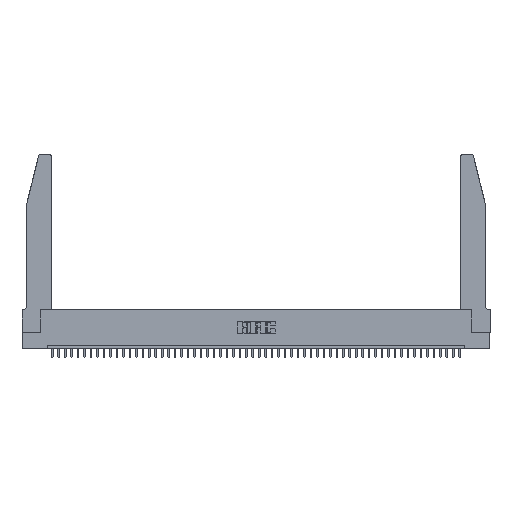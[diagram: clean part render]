
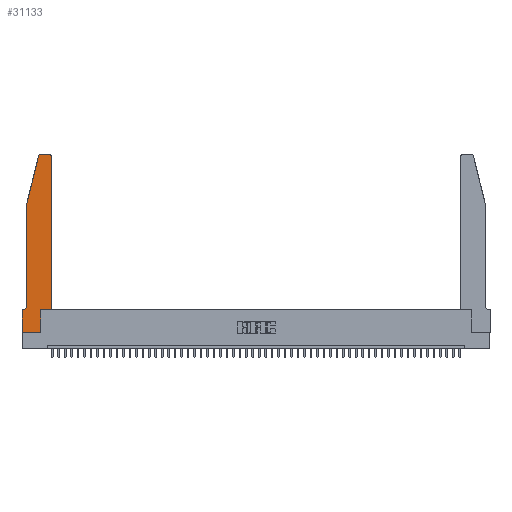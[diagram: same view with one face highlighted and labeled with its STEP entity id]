
A CAD part, top view. The second image highlights one B-rep face of the part: STEP entity #31133.
In plain terms, the highlighted planar face has unit normal (0, 0, 1).
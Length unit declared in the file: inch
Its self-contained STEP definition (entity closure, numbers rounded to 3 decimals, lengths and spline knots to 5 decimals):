
#1717 = ORIENTED_EDGE ( 'NONE', *, *, #28903, .T. ) ;
#1840 = EDGE_CURVE ( 'NONE', #20062, #29995, #32246, .T. ) ;
#2318 = CARTESIAN_POINT ( 'NONE',  ( 0.0055, 0.35, 0.37 ) ) ;
#3267 = CARTESIAN_POINT ( 'NONE',  ( 0.284, 2.75, 0.37 ) ) ;
#3739 = VERTEX_POINT ( 'NONE', #6197 ) ;
#4119 = EDGE_CURVE ( 'NONE', #8806, #45292, #38671, .T. ) ;
#4147 = ORIENTED_EDGE ( 'NONE', *, *, #32344, .T. ) ;
#6197 = CARTESIAN_POINT ( 'NONE',  ( 0., 0.35, 0.37 ) ) ;
#6241 = CARTESIAN_POINT ( 'NONE',  ( 0.25487, 2.72718, 0.37 ) ) ;
#6331 = CARTESIAN_POINT ( 'NONE',  ( 0.4505, 0.35, 0.37 ) ) ;
#6608 = ORIENTED_EDGE ( 'NONE', *, *, #1840, .T. ) ;
#6684 = DIRECTION ( 'NONE',  ( 1., 0., 0. ) ) ;
#6787 = CARTESIAN_POINT ( 'NONE',  ( 0.2605, 2.75, 0.37 ) ) ;
#7058 = CARTESIAN_POINT ( 'NONE',  ( 0.0755, 2., 0.37 ) ) ;
#7132 = AXIS2_PLACEMENT_3D ( 'NONE', #12998, #8782, #47065 ) ;
#7313 = CARTESIAN_POINT ( 'NONE',  ( 0.0755, 2., 0.37 ) ) ;
#7950 = VERTEX_POINT ( 'NONE', #2318 ) ;
#8351 = EDGE_CURVE ( 'NONE', #29320, #8806, #15928, .T. ) ;
#8782 = DIRECTION ( 'NONE',  ( 0., 0., 1. ) ) ;
#8806 = VERTEX_POINT ( 'NONE', #7058 ) ;
#8993 = VERTEX_POINT ( 'NONE', #33100 ) ;
#9275 = CIRCLE ( 'NONE', #34015, 0.07 ) ;
#9447 = CARTESIAN_POINT ( 'NONE',  ( 0.2865, 0., 0.37 ) ) ;
#9483 = VERTEX_POINT ( 'NONE', #9447 ) ;
#9881 = LINE ( 'NONE', #36687, #21960 ) ;
#9987 = CARTESIAN_POINT ( 'NONE',  ( 0.4205, 2.75, 0.37 ) ) ;
#10151 = ORIENTED_EDGE ( 'NONE', *, *, #30791, .T. ) ;
#10547 = ORIENTED_EDGE ( 'NONE', *, *, #25583, .T. ) ;
#11355 = CARTESIAN_POINT ( 'NONE',  ( 0.0755, 2., 0.37 ) ) ;
#12998 = CARTESIAN_POINT ( 'NONE',  ( 0.284, 2.72, 0.37 ) ) ;
#13237 = CARTESIAN_POINT ( 'NONE',  ( 0.4205, 2.72, 0.37 ) ) ;
#13530 = VECTOR ( 'NONE', #30521, 39.37008 ) ;
#14229 = CARTESIAN_POINT ( 'NONE',  ( 0., 0., 0.37 ) ) ;
#15154 = VECTOR ( 'NONE', #26376, 39.37008 ) ;
#15187 = VERTEX_POINT ( 'NONE', #35329 ) ;
#15651 = DIRECTION ( 'NONE',  ( -1., 0., 0. ) ) ;
#15928 = LINE ( 'NONE', #7313, #49155 ) ;
#16139 = VECTOR ( 'NONE', #41015, 39.37008 ) ;
#16503 = LINE ( 'NONE', #6787, #37031 ) ;
#17636 = AXIS2_PLACEMENT_3D ( 'NONE', #13237, #41236, #44765 ) ;
#17648 = CARTESIAN_POINT ( 'NONE',  ( 0.2865, 0.35, 0.37 ) ) ;
#18223 = DIRECTION ( 'NONE',  ( 1., 0., 0. ) ) ;
#19315 = LINE ( 'NONE', #14229, #22286 ) ;
#19633 = CIRCLE ( 'NONE', #17636, 0.03 ) ;
#20062 = VERTEX_POINT ( 'NONE', #17648 ) ;
#20151 = CARTESIAN_POINT ( 'NONE',  ( 0.2865, 0.35, 0.37 ) ) ;
#21692 = ORIENTED_EDGE ( 'NONE', *, *, #29988, .T. ) ;
#21960 = VECTOR ( 'NONE', #40529, 39.37008 ) ;
#22286 = VECTOR ( 'NONE', #6684, 39.37008 ) ;
#25583 = EDGE_CURVE ( 'NONE', #45292, #7950, #9275, .T. ) ;
#25786 = EDGE_CURVE ( 'NONE', #47576, #32890, #16503, .T. ) ;
#26376 = DIRECTION ( 'NONE',  ( -1., 0., 0. ) ) ;
#26380 = CARTESIAN_POINT ( 'NONE',  ( 0., 0., 0.37 ) ) ;
#26384 = CIRCLE ( 'NONE', #7132, 0.03 ) ;
#27130 = VECTOR ( 'NONE', #45809, 39.37008 ) ;
#27507 = ORIENTED_EDGE ( 'NONE', *, *, #8351, .T. ) ;
#27752 = EDGE_CURVE ( 'NONE', #3739, #15187, #35530, .T. ) ;
#27786 = ORIENTED_EDGE ( 'NONE', *, *, #4119, .T. ) ;
#28111 = CARTESIAN_POINT ( 'NONE',  ( 0., 0.35, 0.37 ) ) ;
#28282 = PLANE ( 'NONE',  #44955 ) ;
#28682 = CARTESIAN_POINT ( 'NONE',  ( 0.0755, 0.35, 0.37 ) ) ;
#28903 = EDGE_CURVE ( 'NONE', #15187, #9483, #19315, .T. ) ;
#29320 = VERTEX_POINT ( 'NONE', #6241 ) ;
#29988 = EDGE_CURVE ( 'NONE', #32890, #29320, #26384, .T. ) ;
#29995 = VERTEX_POINT ( 'NONE', #6331 ) ;
#30521 = DIRECTION ( 'NONE',  ( 1., 0., 0. ) ) ;
#30791 = EDGE_CURVE ( 'NONE', #29995, #8993, #9881, .T. ) ;
#31133 = ADVANCED_FACE ( 'NONE', ( #43573 ), #28282, .T. ) ;
#32246 = LINE ( 'NONE', #40028, #13530 ) ;
#32344 = EDGE_CURVE ( 'NONE', #7950, #3739, #36839, .T. ) ;
#32890 = VERTEX_POINT ( 'NONE', #3267 ) ;
#33100 = CARTESIAN_POINT ( 'NONE',  ( 0.4505, 2.72, 0.37 ) ) ;
#34015 = AXIS2_PLACEMENT_3D ( 'NONE', #45849, #37598, #49751 ) ;
#34985 = ORIENTED_EDGE ( 'NONE', *, *, #35623, .T. ) ;
#35026 = CARTESIAN_POINT ( 'NONE',  ( 0.0755, 0.42, 0.37 ) ) ;
#35329 = CARTESIAN_POINT ( 'NONE',  ( 0., 0., 0.37 ) ) ;
#35530 = LINE ( 'NONE', #26380, #27130 ) ;
#35623 = EDGE_CURVE ( 'NONE', #8993, #47576, #19633, .T. ) ;
#36687 = CARTESIAN_POINT ( 'NONE',  ( 0.4505, 0.35, 0.37 ) ) ;
#36839 = LINE ( 'NONE', #28682, #15154 ) ;
#37031 = VECTOR ( 'NONE', #15651, 39.37008 ) ;
#37261 = ORIENTED_EDGE ( 'NONE', *, *, #25786, .T. ) ;
#37598 = DIRECTION ( 'NONE',  ( 0., 0., -1. ) ) ;
#38064 = VECTOR ( 'NONE', #45776, 39.37008 ) ;
#38671 = LINE ( 'NONE', #11355, #38064 ) ;
#40028 = CARTESIAN_POINT ( 'NONE',  ( 0.4505, 0.35, 0.37 ) ) ;
#40153 = DIRECTION ( 'NONE',  ( -0.239, -0.971, 0. ) ) ;
#40529 = DIRECTION ( 'NONE',  ( 0., 1., 0. ) ) ;
#41015 = DIRECTION ( 'NONE',  ( 0., 1., 0. ) ) ;
#41054 = EDGE_CURVE ( 'NONE', #9483, #20062, #46906, .T. ) ;
#41236 = DIRECTION ( 'NONE',  ( 0., 0., 1. ) ) ;
#41527 = ORIENTED_EDGE ( 'NONE', *, *, #41054, .T. ) ;
#43573 = FACE_OUTER_BOUND ( 'NONE', #43741, .T. ) ;
#43741 = EDGE_LOOP ( 'NONE', ( #37261, #21692, #27507, #27786, #10547, #4147, #48189, #1717, #41527, #6608, #10151, #34985 ) ) ;
#44461 = DIRECTION ( 'NONE',  ( 0., 0., 1. ) ) ;
#44765 = DIRECTION ( 'NONE',  ( 1., 0., 0. ) ) ;
#44955 = AXIS2_PLACEMENT_3D ( 'NONE', #28111, #44461, #18223 ) ;
#45292 = VERTEX_POINT ( 'NONE', #35026 ) ;
#45776 = DIRECTION ( 'NONE',  ( 0., -1., 0. ) ) ;
#45809 = DIRECTION ( 'NONE',  ( 0., -1., 0. ) ) ;
#45849 = CARTESIAN_POINT ( 'NONE',  ( 0.0055, 0.42, 0.37 ) ) ;
#46906 = LINE ( 'NONE', #20151, #16139 ) ;
#47065 = DIRECTION ( 'NONE',  ( 1., 0., 0. ) ) ;
#47576 = VERTEX_POINT ( 'NONE', #9987 ) ;
#48189 = ORIENTED_EDGE ( 'NONE', *, *, #27752, .T. ) ;
#49155 = VECTOR ( 'NONE', #40153, 39.37008 ) ;
#49751 = DIRECTION ( 'NONE',  ( -1., 0., 0. ) ) ;
